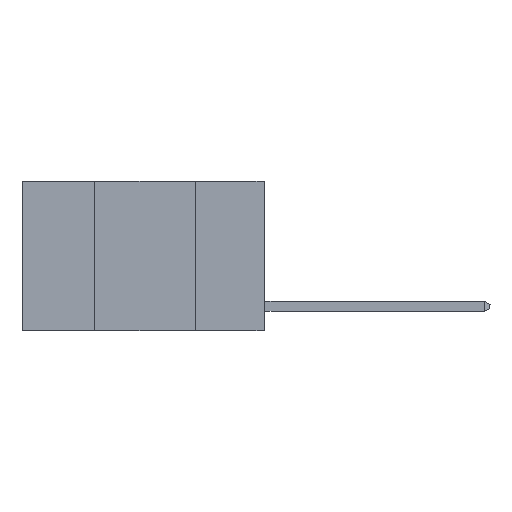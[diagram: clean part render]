
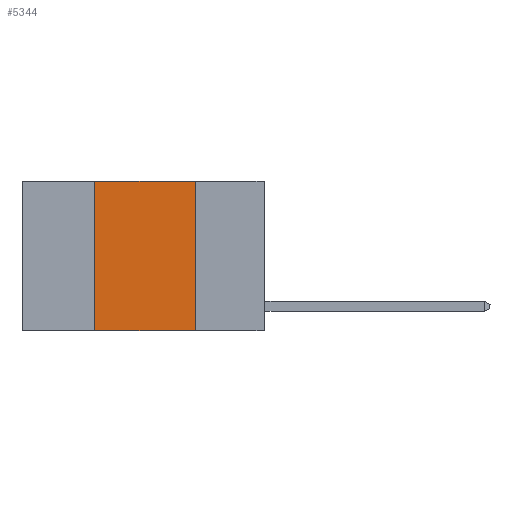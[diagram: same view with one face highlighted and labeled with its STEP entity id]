
A CAD part, left-side view. The second image highlights one B-rep face of the part: STEP entity #5344.
In plain terms, the highlighted planar face has unit normal (-1, 0, 0).
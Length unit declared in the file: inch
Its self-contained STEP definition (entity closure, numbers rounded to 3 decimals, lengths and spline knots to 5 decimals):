
#782 = VECTOR ( 'NONE', #11816, 39.37008 ) ;
#823 = VECTOR ( 'NONE', #18075, 39.37008 ) ;
#1032 = CARTESIAN_POINT ( 'NONE',  ( 0., 0.42, 0. ) ) ;
#1103 = PLANE ( 'NONE',  #21246 ) ;
#1337 = EDGE_CURVE ( 'NONE', #3929, #7033, #20532, .T. ) ;
#1546 = EDGE_CURVE ( 'NONE', #12229, #21411, #5768, .T. ) ;
#1644 = DIRECTION ( 'NONE',  ( 0., -1., 0. ) ) ;
#1950 = EDGE_CURVE ( 'NONE', #7033, #21411, #10449, .T. ) ;
#2923 = DIRECTION ( 'NONE',  ( 0., 0., -1. ) ) ;
#3066 = CARTESIAN_POINT ( 'NONE',  ( 0., 0.6, 0. ) ) ;
#3929 = VERTEX_POINT ( 'NONE', #12710 ) ;
#4372 = CARTESIAN_POINT ( 'NONE',  ( 0., 0.6, 0. ) ) ;
#5344 = ADVANCED_FACE ( 'NONE', ( #21452 ), #1103, .F. ) ;
#5475 = ORIENTED_EDGE ( 'NONE', *, *, #7171, .F. ) ;
#5538 = ORIENTED_EDGE ( 'NONE', *, *, #1337, .F. ) ;
#5768 = LINE ( 'NONE', #12103, #782 ) ;
#6801 = VECTOR ( 'NONE', #20486, 39.37008 ) ;
#7014 = CARTESIAN_POINT ( 'NONE',  ( 0., 0.17, 0. ) ) ;
#7033 = VERTEX_POINT ( 'NONE', #8662 ) ;
#7171 = EDGE_CURVE ( 'NONE', #12229, #3929, #14475, .T. ) ;
#8662 = CARTESIAN_POINT ( 'NONE',  ( 0., 0.17, 0. ) ) ;
#9177 = VECTOR ( 'NONE', #1644, 39.37008 ) ;
#10449 = LINE ( 'NONE', #7014, #6801 ) ;
#10524 = CARTESIAN_POINT ( 'NONE',  ( 0., 0.42, -0.37 ) ) ;
#11816 = DIRECTION ( 'NONE',  ( 0., -1., 0. ) ) ;
#12103 = CARTESIAN_POINT ( 'NONE',  ( 0., 0.6, -0.37 ) ) ;
#12229 = VERTEX_POINT ( 'NONE', #10524 ) ;
#12710 = CARTESIAN_POINT ( 'NONE',  ( 0., 0.42, 0. ) ) ;
#12876 = ORIENTED_EDGE ( 'NONE', *, *, #1950, .F. ) ;
#14475 = LINE ( 'NONE', #1032, #823 ) ;
#18075 = DIRECTION ( 'NONE',  ( 0., 0., 1. ) ) ;
#18991 = ORIENTED_EDGE ( 'NONE', *, *, #1546, .T. ) ;
#20486 = DIRECTION ( 'NONE',  ( 0., 0., -1. ) ) ;
#20532 = LINE ( 'NONE', #4372, #9177 ) ;
#20824 = EDGE_LOOP ( 'NONE', ( #12876, #5538, #5475, #18991 ) ) ;
#21246 = AXIS2_PLACEMENT_3D ( 'NONE', #3066, #21279, #2923 ) ;
#21279 = DIRECTION ( 'NONE',  ( 1., 0., 0. ) ) ;
#21411 = VERTEX_POINT ( 'NONE', #21608 ) ;
#21452 = FACE_OUTER_BOUND ( 'NONE', #20824, .T. ) ;
#21608 = CARTESIAN_POINT ( 'NONE',  ( 0., 0.17, -0.37 ) ) ;
